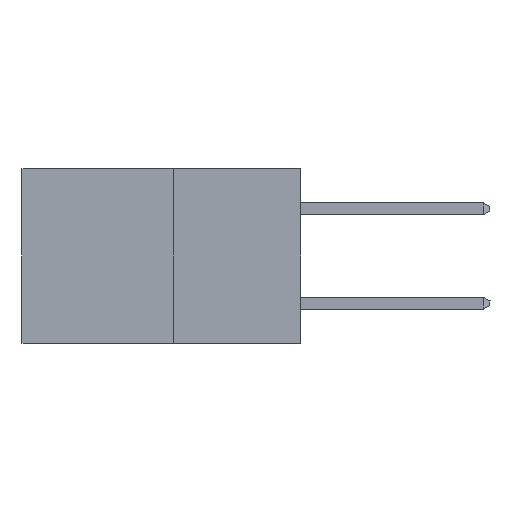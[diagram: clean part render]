
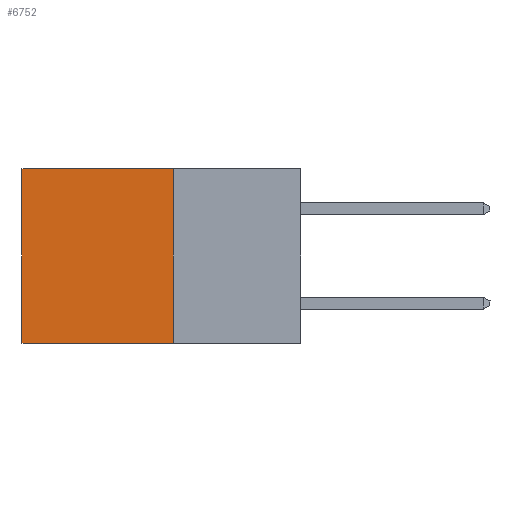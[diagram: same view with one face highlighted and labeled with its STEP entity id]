
A CAD part, left-side view. The second image highlights one B-rep face of the part: STEP entity #6752.
In plain terms, the highlighted planar face has unit normal (-1, 0, 0).
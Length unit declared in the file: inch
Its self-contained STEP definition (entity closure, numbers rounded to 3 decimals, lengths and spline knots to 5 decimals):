
#227 = VECTOR ( 'NONE', #6943, 39.37008 ) ;
#864 = VECTOR ( 'NONE', #8642, 39.37008 ) ;
#1294 = EDGE_CURVE ( 'NONE', #1627, #6232, #6945, .T. ) ;
#1323 = CARTESIAN_POINT ( 'NONE',  ( 0.277, 0.27, 0. ) ) ;
#1627 = VERTEX_POINT ( 'NONE', #1323 ) ;
#2321 = ORIENTED_EDGE ( 'NONE', *, *, #1294, .F. ) ;
#2460 = CARTESIAN_POINT ( 'NONE',  ( 0.277, 0.59, 0. ) ) ;
#2473 = VERTEX_POINT ( 'NONE', #2460 ) ;
#2744 = EDGE_CURVE ( 'NONE', #6232, #6233, #4595, .T. ) ;
#2818 = DIRECTION ( 'NONE',  ( 0., 0., -1. ) ) ;
#2980 = CARTESIAN_POINT ( 'NONE',  ( 0.277, 0.27, -0.37 ) ) ;
#3089 = VECTOR ( 'NONE', #2818, 39.37008 ) ;
#3143 = AXIS2_PLACEMENT_3D ( 'NONE', #6382, #6164, #6112 ) ;
#3391 = VECTOR ( 'NONE', #5680, 39.37008 ) ;
#3397 = EDGE_CURVE ( 'NONE', #2473, #6233, #7010, .T. ) ;
#3628 = CARTESIAN_POINT ( 'NONE',  ( 0.277, 0.27, -0.37 ) ) ;
#4595 = LINE ( 'NONE', #3628, #227 ) ;
#4951 = CARTESIAN_POINT ( 'NONE',  ( 0.277, 0.59, -0.37 ) ) ;
#5109 = CARTESIAN_POINT ( 'NONE',  ( 0.277, 0.59, -0.37 ) ) ;
#5680 = DIRECTION ( 'NONE',  ( 0., 0., -1. ) ) ;
#5851 = FACE_OUTER_BOUND ( 'NONE', #7459, .T. ) ;
#5864 = CARTESIAN_POINT ( 'NONE',  ( 0.277, 0.27, -0.37 ) ) ;
#6112 = DIRECTION ( 'NONE',  ( 0., 0., -1. ) ) ;
#6127 = ORIENTED_EDGE ( 'NONE', *, *, #8692, .T. ) ;
#6164 = DIRECTION ( 'NONE',  ( 1., 0., 0. ) ) ;
#6232 = VERTEX_POINT ( 'NONE', #5864 ) ;
#6233 = VERTEX_POINT ( 'NONE', #4951 ) ;
#6382 = CARTESIAN_POINT ( 'NONE',  ( 0.277, 0.27, -0.37 ) ) ;
#6418 = PLANE ( 'NONE',  #3143 ) ;
#6454 = CARTESIAN_POINT ( 'NONE',  ( 0.277, 0.27, 0. ) ) ;
#6752 = ADVANCED_FACE ( 'NONE', ( #5851 ), #6418, .F. ) ;
#6943 = DIRECTION ( 'NONE',  ( 0., 1., 0. ) ) ;
#6945 = LINE ( 'NONE', #2980, #3089 ) ;
#7010 = LINE ( 'NONE', #5109, #3391 ) ;
#7029 = LINE ( 'NONE', #6454, #864 ) ;
#7459 = EDGE_LOOP ( 'NONE', ( #8463, #8815, #2321, #6127 ) ) ;
#8463 = ORIENTED_EDGE ( 'NONE', *, *, #3397, .T. ) ;
#8642 = DIRECTION ( 'NONE',  ( 0., 1., 0. ) ) ;
#8692 = EDGE_CURVE ( 'NONE', #1627, #2473, #7029, .T. ) ;
#8815 = ORIENTED_EDGE ( 'NONE', *, *, #2744, .F. ) ;
